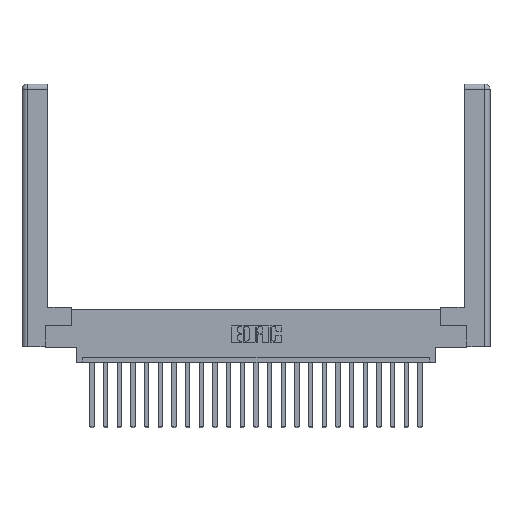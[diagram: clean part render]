
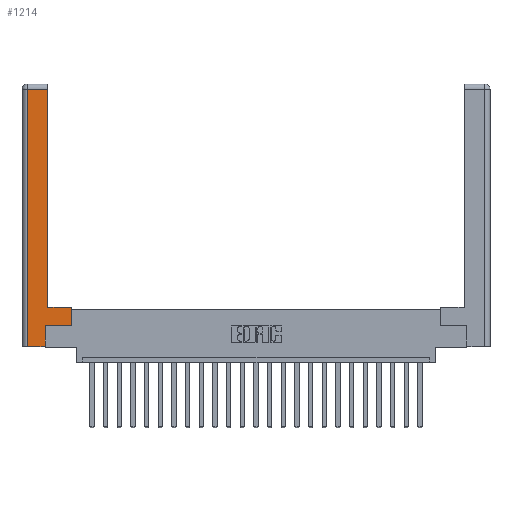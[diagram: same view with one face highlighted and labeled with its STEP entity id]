
A CAD part, top view. The second image highlights one B-rep face of the part: STEP entity #1214.
In plain terms, the highlighted planar face has unit normal (0, 0, 1).
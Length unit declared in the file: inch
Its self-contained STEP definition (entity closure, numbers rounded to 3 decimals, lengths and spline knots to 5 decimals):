
#526 = EDGE_CURVE ( 'NONE', #10537, #15290, #13781, .T. ) ;
#660 = VERTEX_POINT ( 'NONE', #6662 ) ;
#724 = CARTESIAN_POINT ( 'NONE',  ( 0.265, 0.245, 0. ) ) ;
#1188 = VERTEX_POINT ( 'NONE', #12155 ) ;
#1214 = ADVANCED_FACE ( 'NONE', ( #11195 ), #22788, .F. ) ;
#1301 = CARTESIAN_POINT ( 'NONE',  ( 0.295, 0.45, 0. ) ) ;
#2477 = VECTOR ( 'NONE', #13389, 39.37008 ) ;
#2950 = EDGE_CURVE ( 'NONE', #12499, #14485, #16613, .T. ) ;
#3106 = CARTESIAN_POINT ( 'NONE',  ( 0.265, 0., 0. ) ) ;
#3776 = DIRECTION ( 'NONE',  ( 1., 0., 0. ) ) ;
#4177 = EDGE_CURVE ( 'NONE', #22200, #12499, #10693, .T. ) ;
#4297 = LINE ( 'NONE', #3106, #8537 ) ;
#4551 = CARTESIAN_POINT ( 'NONE',  ( 0.0615, 2.94, 0. ) ) ;
#5519 = EDGE_LOOP ( 'NONE', ( #10039, #14534, #15339, #13910, #6991, #7213, #17552, #13787 ) ) ;
#6662 = CARTESIAN_POINT ( 'NONE',  ( 0.265, 0., 0. ) ) ;
#6694 = VECTOR ( 'NONE', #10321, 39.37008 ) ;
#6903 = CARTESIAN_POINT ( 'NONE',  ( 0.565, 0.45, 0. ) ) ;
#6991 = ORIENTED_EDGE ( 'NONE', *, *, #23267, .T. ) ;
#7213 = ORIENTED_EDGE ( 'NONE', *, *, #7794, .T. ) ;
#7254 = CARTESIAN_POINT ( 'NONE',  ( 0.0615, 0., 0. ) ) ;
#7794 = EDGE_CURVE ( 'NONE', #11251, #1188, #17532, .T. ) ;
#7810 = LINE ( 'NONE', #6903, #6694 ) ;
#8229 = DIRECTION ( 'NONE',  ( 1., 0., 0. ) ) ;
#8537 = VECTOR ( 'NONE', #3776, 39.37008 ) ;
#9077 = AXIS2_PLACEMENT_3D ( 'NONE', #13907, #15573, #15799 ) ;
#9104 = VECTOR ( 'NONE', #20491, 39.37008 ) ;
#9390 = CARTESIAN_POINT ( 'NONE',  ( 0.295, 0.45, 0. ) ) ;
#9607 = VECTOR ( 'NONE', #8229, 39.37008 ) ;
#9913 = CARTESIAN_POINT ( 'NONE',  ( 0.295, 3., 0. ) ) ;
#10039 = ORIENTED_EDGE ( 'NONE', *, *, #2950, .T. ) ;
#10321 = DIRECTION ( 'NONE',  ( 0., 1., 0. ) ) ;
#10537 = VERTEX_POINT ( 'NONE', #12479 ) ;
#10693 = LINE ( 'NONE', #9390, #23082 ) ;
#11195 = FACE_OUTER_BOUND ( 'NONE', #5519, .T. ) ;
#11196 = LINE ( 'NONE', #4551, #18246 ) ;
#11234 = VECTOR ( 'NONE', #15270, 39.37008 ) ;
#11251 = VERTEX_POINT ( 'NONE', #14583 ) ;
#11782 = CARTESIAN_POINT ( 'NONE',  ( 0.0615, 0., 0. ) ) ;
#12155 = CARTESIAN_POINT ( 'NONE',  ( 0.565, 0.245, 0. ) ) ;
#12479 = CARTESIAN_POINT ( 'NONE',  ( 0.0615, 2.94, 0. ) ) ;
#12499 = VERTEX_POINT ( 'NONE', #1301 ) ;
#12963 = EDGE_CURVE ( 'NONE', #15290, #660, #4297, .T. ) ;
#13291 = DIRECTION ( 'NONE',  ( -1., 0., 0. ) ) ;
#13389 = DIRECTION ( 'NONE',  ( 0., 1., 0. ) ) ;
#13601 = CARTESIAN_POINT ( 'NONE',  ( 0.565, 0.245, 0. ) ) ;
#13781 = LINE ( 'NONE', #11782, #11234 ) ;
#13787 = ORIENTED_EDGE ( 'NONE', *, *, #4177, .T. ) ;
#13907 = CARTESIAN_POINT ( 'NONE',  ( 0., 0., 0. ) ) ;
#13910 = ORIENTED_EDGE ( 'NONE', *, *, #12963, .T. ) ;
#14485 = VERTEX_POINT ( 'NONE', #17180 ) ;
#14534 = ORIENTED_EDGE ( 'NONE', *, *, #20782, .T. ) ;
#14583 = CARTESIAN_POINT ( 'NONE',  ( 0.265, 0.245, 0. ) ) ;
#14771 = DIRECTION ( 'NONE',  ( -1., 0., 0. ) ) ;
#15270 = DIRECTION ( 'NONE',  ( 0., -1., 0. ) ) ;
#15290 = VERTEX_POINT ( 'NONE', #7254 ) ;
#15339 = ORIENTED_EDGE ( 'NONE', *, *, #526, .T. ) ;
#15573 = DIRECTION ( 'NONE',  ( 0., 0., -1. ) ) ;
#15799 = DIRECTION ( 'NONE',  ( -1., 0., 0. ) ) ;
#16613 = LINE ( 'NONE', #9913, #2477 ) ;
#17180 = CARTESIAN_POINT ( 'NONE',  ( 0.295, 2.94, 0. ) ) ;
#17532 = LINE ( 'NONE', #13601, #9607 ) ;
#17552 = ORIENTED_EDGE ( 'NONE', *, *, #18256, .T. ) ;
#18123 = LINE ( 'NONE', #724, #9104 ) ;
#18246 = VECTOR ( 'NONE', #13291, 39.37008 ) ;
#18256 = EDGE_CURVE ( 'NONE', #1188, #22200, #7810, .T. ) ;
#20491 = DIRECTION ( 'NONE',  ( 0., 1., 0. ) ) ;
#20782 = EDGE_CURVE ( 'NONE', #14485, #10537, #11196, .T. ) ;
#22200 = VERTEX_POINT ( 'NONE', #23042 ) ;
#22788 = PLANE ( 'NONE',  #9077 ) ;
#23042 = CARTESIAN_POINT ( 'NONE',  ( 0.565, 0.45, 0. ) ) ;
#23082 = VECTOR ( 'NONE', #14771, 39.37008 ) ;
#23267 = EDGE_CURVE ( 'NONE', #660, #11251, #18123, .T. ) ;
